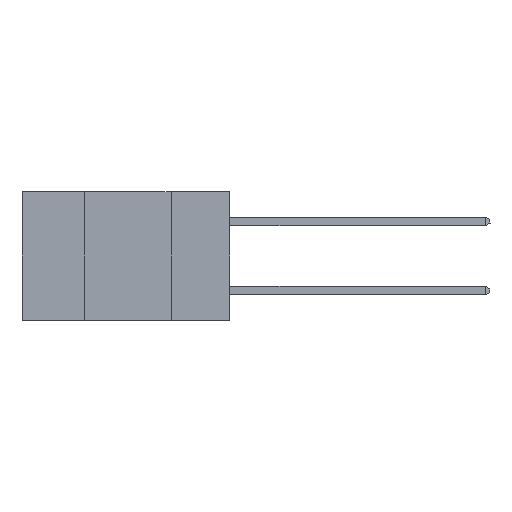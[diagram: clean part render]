
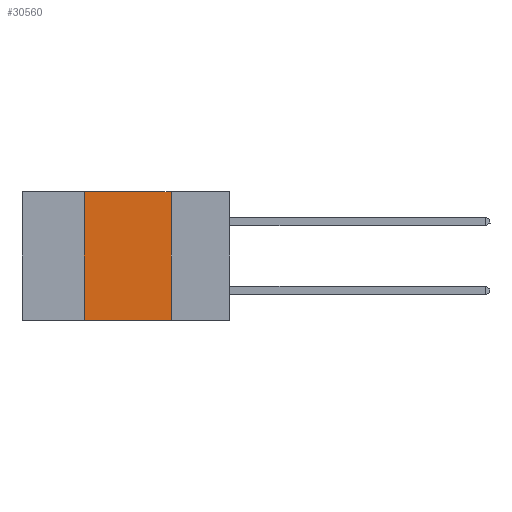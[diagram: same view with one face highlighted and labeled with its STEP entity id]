
A CAD part, left-side view. The second image highlights one B-rep face of the part: STEP entity #30560.
In plain terms, the highlighted planar face has unit normal (-1, 0, 0).
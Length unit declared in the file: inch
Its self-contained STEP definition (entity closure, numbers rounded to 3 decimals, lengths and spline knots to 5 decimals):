
#903 = VERTEX_POINT ( 'NONE', #14002 ) ;
#1495 = CARTESIAN_POINT ( 'NONE',  ( 0., 0.6, -0.37 ) ) ;
#2931 = CARTESIAN_POINT ( 'NONE',  ( 0., 0.6, 0. ) ) ;
#4847 = EDGE_CURVE ( 'NONE', #24705, #18997, #22312, .T. ) ;
#6101 = AXIS2_PLACEMENT_3D ( 'NONE', #11853, #30065, #14462 ) ;
#6617 = PLANE ( 'NONE',  #6101 ) ;
#6821 = CARTESIAN_POINT ( 'NONE',  ( 0., 0.17, -0.37 ) ) ;
#7108 = CARTESIAN_POINT ( 'NONE',  ( 0., 0.42, -0.37 ) ) ;
#7623 = CARTESIAN_POINT ( 'NONE',  ( 0., 0.17, 0. ) ) ;
#8418 = DIRECTION ( 'NONE',  ( 0., 0., 1. ) ) ;
#8612 = LINE ( 'NONE', #31175, #30213 ) ;
#11295 = ORIENTED_EDGE ( 'NONE', *, *, #17286, .F. ) ;
#11853 = CARTESIAN_POINT ( 'NONE',  ( 0., 0.6, 0. ) ) ;
#12583 = VECTOR ( 'NONE', #8418, 39.37008 ) ;
#13073 = DIRECTION ( 'NONE',  ( 0., 0., -1. ) ) ;
#13402 = LINE ( 'NONE', #21450, #12583 ) ;
#14002 = CARTESIAN_POINT ( 'NONE',  ( 0., 0.42, 0. ) ) ;
#14462 = DIRECTION ( 'NONE',  ( 0., 0., -1. ) ) ;
#16185 = LINE ( 'NONE', #2931, #29237 ) ;
#17286 = EDGE_CURVE ( 'NONE', #903, #21290, #16185, .T. ) ;
#17808 = ORIENTED_EDGE ( 'NONE', *, *, #27430, .F. ) ;
#18997 = VERTEX_POINT ( 'NONE', #6821 ) ;
#19655 = EDGE_LOOP ( 'NONE', ( #30027, #11295, #17808, #28439 ) ) ;
#21290 = VERTEX_POINT ( 'NONE', #7623 ) ;
#21450 = CARTESIAN_POINT ( 'NONE',  ( 0., 0.42, 0. ) ) ;
#22312 = LINE ( 'NONE', #1495, #28387 ) ;
#24705 = VERTEX_POINT ( 'NONE', #7108 ) ;
#25599 = EDGE_CURVE ( 'NONE', #21290, #18997, #8612, .T. ) ;
#27430 = EDGE_CURVE ( 'NONE', #24705, #903, #13402, .T. ) ;
#28387 = VECTOR ( 'NONE', #30217, 39.37008 ) ;
#28439 = ORIENTED_EDGE ( 'NONE', *, *, #4847, .T. ) ;
#28884 = DIRECTION ( 'NONE',  ( 0., -1., 0. ) ) ;
#29237 = VECTOR ( 'NONE', #28884, 39.37008 ) ;
#30027 = ORIENTED_EDGE ( 'NONE', *, *, #25599, .F. ) ;
#30065 = DIRECTION ( 'NONE',  ( 1., 0., 0. ) ) ;
#30213 = VECTOR ( 'NONE', #13073, 39.37008 ) ;
#30217 = DIRECTION ( 'NONE',  ( 0., -1., 0. ) ) ;
#30560 = ADVANCED_FACE ( 'NONE', ( #31936 ), #6617, .F. ) ;
#31175 = CARTESIAN_POINT ( 'NONE',  ( 0., 0.17, 0. ) ) ;
#31936 = FACE_OUTER_BOUND ( 'NONE', #19655, .T. ) ;
